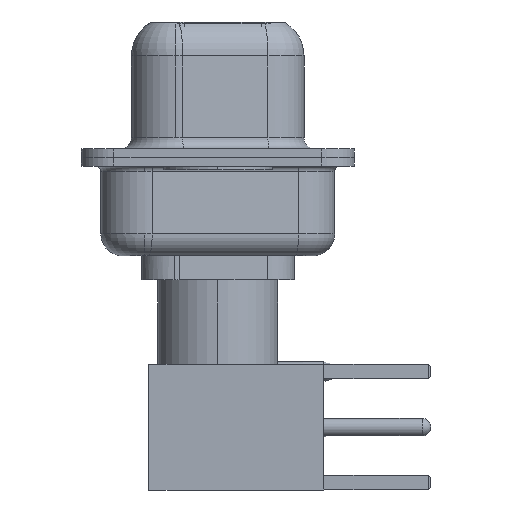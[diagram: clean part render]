
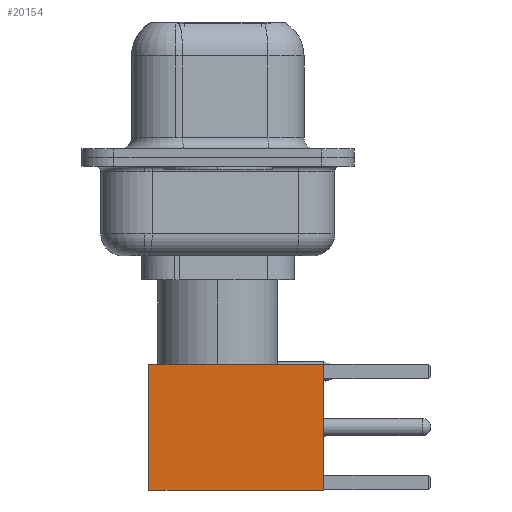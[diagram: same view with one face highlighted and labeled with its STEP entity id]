
A CAD part, left-side view. The second image highlights one B-rep face of the part: STEP entity #20154.
In plain terms, the highlighted face is planar.
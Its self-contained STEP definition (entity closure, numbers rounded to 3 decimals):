
#71 = EDGE_LOOP ( 'NONE', ( #8993, #9941, #11416, #9858 ) ) ;
#218 = DIRECTION ( 'NONE',  ( 0., 0., -1. ) ) ;
#447 = VECTOR ( 'NONE', #634, 1000. ) ;
#634 = DIRECTION ( 'NONE',  ( 0., 0., -1. ) ) ;
#1197 = VECTOR ( 'NONE', #1627, 1000. ) ;
#1627 = DIRECTION ( 'NONE',  ( -1., 0., 0. ) ) ;
#1656 = CARTESIAN_POINT ( 'NONE',  ( 2.875, 2.875, 0. ) ) ;
#1703 = CARTESIAN_POINT ( 'NONE',  ( 0., 2.875, 0. ) ) ;
#2021 = LINE ( 'NONE', #1703, #13624 ) ;
#3339 = DIRECTION ( 'NONE',  ( 0., 1., 0. ) ) ;
#3511 = EDGE_CURVE ( 'NONE', #17304, #4462, #11976, .T. ) ;
#3544 = LINE ( 'NONE', #9691, #1197 ) ;
#4462 = VERTEX_POINT ( 'NONE', #7442 ) ;
#4752 = CARTESIAN_POINT ( 'NONE',  ( -2.875, 2.875, 0. ) ) ;
#4818 = EDGE_CURVE ( 'NONE', #5089, #17125, #14869, .T. ) ;
#5089 = VERTEX_POINT ( 'NONE', #17498 ) ;
#5385 = CARTESIAN_POINT ( 'NONE',  ( 2.875, 2.875, 8. ) ) ;
#7442 = CARTESIAN_POINT ( 'NONE',  ( 2.875, 2.875, 0. ) ) ;
#7597 = VECTOR ( 'NONE', #218, 1000. ) ;
#8993 = ORIENTED_EDGE ( 'NONE', *, *, #3511, .T. ) ;
#9691 = CARTESIAN_POINT ( 'NONE',  ( 0., 2.875, 8. ) ) ;
#9715 = PLANE ( 'NONE',  #10023 ) ;
#9858 = ORIENTED_EDGE ( 'NONE', *, *, #19375, .F. ) ;
#9941 = ORIENTED_EDGE ( 'NONE', *, *, #16709, .T. ) ;
#10023 = AXIS2_PLACEMENT_3D ( 'NONE', #1656, #3339, #19696 ) ;
#10392 = CARTESIAN_POINT ( 'NONE',  ( 2.875, 2.875, 0. ) ) ;
#11416 = ORIENTED_EDGE ( 'NONE', *, *, #4818, .F. ) ;
#11557 = DIRECTION ( 'NONE',  ( -1., 0., 0. ) ) ;
#11976 = LINE ( 'NONE', #10392, #447 ) ;
#13624 = VECTOR ( 'NONE', #11557, 1000. ) ;
#14869 = LINE ( 'NONE', #19746, #7597 ) ;
#15968 = FACE_OUTER_BOUND ( 'NONE', #71, .T. ) ;
#16709 = EDGE_CURVE ( 'NONE', #4462, #17125, #2021, .T. ) ;
#17125 = VERTEX_POINT ( 'NONE', #4752 ) ;
#17304 = VERTEX_POINT ( 'NONE', #5385 ) ;
#17498 = CARTESIAN_POINT ( 'NONE',  ( -2.875, 2.875, 8. ) ) ;
#19375 = EDGE_CURVE ( 'NONE', #17304, #5089, #3544, .T. ) ;
#19696 = DIRECTION ( 'NONE',  ( 0., 0., 1. ) ) ;
#19746 = CARTESIAN_POINT ( 'NONE',  ( -2.875, 2.875, 0. ) ) ;
#20154 = ADVANCED_FACE ( 'NONE', ( #15968 ), #9715, .T. ) ;
